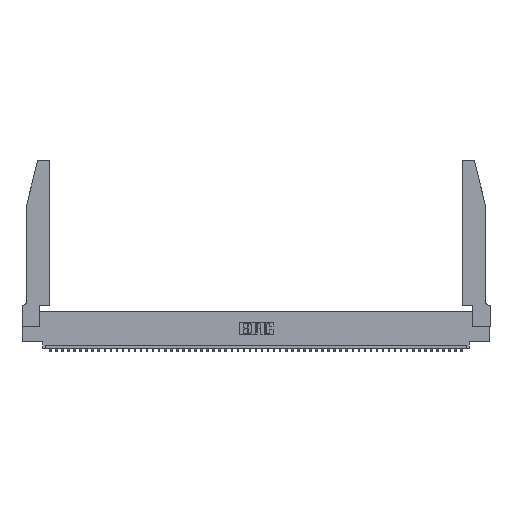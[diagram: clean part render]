
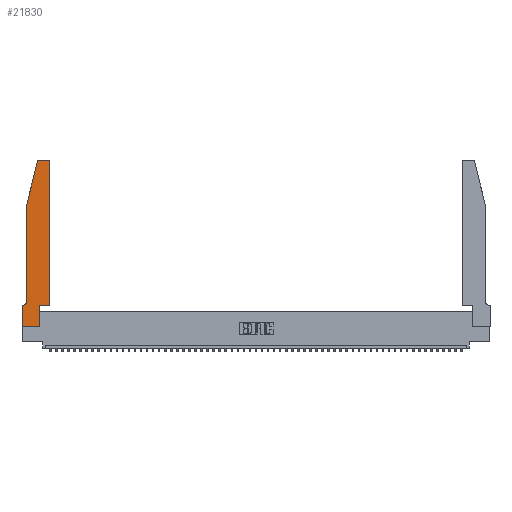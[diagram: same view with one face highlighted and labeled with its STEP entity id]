
A CAD part, top view. The second image highlights one B-rep face of the part: STEP entity #21830.
In plain terms, the highlighted planar face has unit normal (0, 0, 1).
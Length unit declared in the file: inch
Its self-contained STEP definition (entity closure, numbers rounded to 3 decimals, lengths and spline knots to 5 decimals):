
#239 = LINE ( 'NONE', #25851, #21448 ) ;
#1232 = CARTESIAN_POINT ( 'NONE',  ( 0., 0., 0.37 ) ) ;
#1386 = DIRECTION ( 'NONE',  ( 0., 0., 1. ) ) ;
#2253 = VERTEX_POINT ( 'NONE', #44497 ) ;
#3113 = VECTOR ( 'NONE', #41160, 39.37008 ) ;
#3947 = VECTOR ( 'NONE', #29542, 39.37008 ) ;
#3979 = LINE ( 'NONE', #7319, #29633 ) ;
#4258 = EDGE_CURVE ( 'NONE', #22931, #20727, #239, .T. ) ;
#4473 = ORIENTED_EDGE ( 'NONE', *, *, #10888, .T. ) ;
#4487 = CARTESIAN_POINT ( 'NONE',  ( 0.4505, 2.72, 0.37 ) ) ;
#5545 = CARTESIAN_POINT ( 'NONE',  ( 0.4205, 2.72, 0.37 ) ) ;
#6662 = EDGE_CURVE ( 'NONE', #20727, #7962, #49539, .T. ) ;
#7319 = CARTESIAN_POINT ( 'NONE',  ( 0.4505, 0.35, 0.37 ) ) ;
#7406 = VERTEX_POINT ( 'NONE', #10299 ) ;
#7962 = VERTEX_POINT ( 'NONE', #19062 ) ;
#8194 = ORIENTED_EDGE ( 'NONE', *, *, #32107, .T. ) ;
#8564 = LINE ( 'NONE', #29161, #27917 ) ;
#8769 = LINE ( 'NONE', #27854, #45506 ) ;
#9931 = EDGE_LOOP ( 'NONE', ( #43637, #41427, #31588, #38553, #4473, #43729, #26091, #50199, #17724, #44850, #39837, #8194 ) ) ;
#10299 = CARTESIAN_POINT ( 'NONE',  ( 0.25487, 2.72718, 0.37 ) ) ;
#10380 = VERTEX_POINT ( 'NONE', #24235 ) ;
#10888 = EDGE_CURVE ( 'NONE', #23437, #10380, #26225, .T. ) ;
#13756 = CARTESIAN_POINT ( 'NONE',  ( 0.0055, 0.42, 0.37 ) ) ;
#14034 = AXIS2_PLACEMENT_3D ( 'NONE', #5545, #1386, #48073 ) ;
#15065 = DIRECTION ( 'NONE',  ( 1., 0., 0. ) ) ;
#15107 = CARTESIAN_POINT ( 'NONE',  ( 0.4205, 2.75, 0.37 ) ) ;
#16115 = EDGE_CURVE ( 'NONE', #27870, #21726, #28278, .T. ) ;
#17018 = CARTESIAN_POINT ( 'NONE',  ( 0.2605, 2.75, 0.37 ) ) ;
#17303 = LINE ( 'NONE', #1232, #3947 ) ;
#17724 = ORIENTED_EDGE ( 'NONE', *, *, #6662, .T. ) ;
#18154 = AXIS2_PLACEMENT_3D ( 'NONE', #43521, #31065, #35244 ) ;
#19062 = CARTESIAN_POINT ( 'NONE',  ( 0.2865, 0.35, 0.37 ) ) ;
#19545 = DIRECTION ( 'NONE',  ( 0., 0., -1. ) ) ;
#19902 = EDGE_CURVE ( 'NONE', #7962, #46887, #3979, .T. ) ;
#20701 = AXIS2_PLACEMENT_3D ( 'NONE', #37702, #41844, #42013 ) ;
#20727 = VERTEX_POINT ( 'NONE', #30336 ) ;
#21448 = VECTOR ( 'NONE', #39375, 39.37008 ) ;
#21481 = CIRCLE ( 'NONE', #14034, 0.03 ) ;
#21726 = VERTEX_POINT ( 'NONE', #35262 ) ;
#21830 = ADVANCED_FACE ( 'NONE', ( #52040 ), #37760, .T. ) ;
#22159 = CARTESIAN_POINT ( 'NONE',  ( 0.0755, 2., 0.37 ) ) ;
#22931 = VERTEX_POINT ( 'NONE', #35348 ) ;
#23029 = AXIS2_PLACEMENT_3D ( 'NONE', #13756, #19545, #42838 ) ;
#23339 = EDGE_CURVE ( 'NONE', #7406, #36113, #36553, .T. ) ;
#23405 = EDGE_CURVE ( 'NONE', #10380, #2253, #8769, .T. ) ;
#23437 = VERTEX_POINT ( 'NONE', #53276 ) ;
#24235 = CARTESIAN_POINT ( 'NONE',  ( 0.0055, 0.35, 0.37 ) ) ;
#25851 = CARTESIAN_POINT ( 'NONE',  ( 0., 0., 0.37 ) ) ;
#26091 = ORIENTED_EDGE ( 'NONE', *, *, #33414, .T. ) ;
#26225 = CIRCLE ( 'NONE', #23029, 0.07 ) ;
#26385 = DIRECTION ( 'NONE',  ( 0., 1., 0. ) ) ;
#27424 = LINE ( 'NONE', #53063, #35157 ) ;
#27854 = CARTESIAN_POINT ( 'NONE',  ( 0.0755, 0.35, 0.37 ) ) ;
#27870 = VERTEX_POINT ( 'NONE', #15107 ) ;
#27917 = VECTOR ( 'NONE', #46079, 39.37008 ) ;
#28278 = LINE ( 'NONE', #17018, #3113 ) ;
#29161 = CARTESIAN_POINT ( 'NONE',  ( 0.0755, 2., 0.37 ) ) ;
#29542 = DIRECTION ( 'NONE',  ( 0., -1., 0. ) ) ;
#29633 = VECTOR ( 'NONE', #15065, 39.37008 ) ;
#30336 = CARTESIAN_POINT ( 'NONE',  ( 0.2865, 0., 0.37 ) ) ;
#31065 = DIRECTION ( 'NONE',  ( 0., 0., 1. ) ) ;
#31588 = ORIENTED_EDGE ( 'NONE', *, *, #23339, .T. ) ;
#32107 = EDGE_CURVE ( 'NONE', #52682, #27870, #21481, .T. ) ;
#32845 = EDGE_CURVE ( 'NONE', #36113, #23437, #8564, .T. ) ;
#33302 = VECTOR ( 'NONE', #38314, 39.37008 ) ;
#33414 = EDGE_CURVE ( 'NONE', #2253, #22931, #17303, .T. ) ;
#33609 = CARTESIAN_POINT ( 'NONE',  ( 0.2865, 0.35, 0.37 ) ) ;
#35157 = VECTOR ( 'NONE', #40979, 39.37008 ) ;
#35244 = DIRECTION ( 'NONE',  ( 1., 0., 0. ) ) ;
#35262 = CARTESIAN_POINT ( 'NONE',  ( 0.284, 2.75, 0.37 ) ) ;
#35348 = CARTESIAN_POINT ( 'NONE',  ( 0., 0., 0.37 ) ) ;
#35590 = CARTESIAN_POINT ( 'NONE',  ( 0.4505, 0.35, 0.37 ) ) ;
#36041 = VECTOR ( 'NONE', #26385, 39.37008 ) ;
#36113 = VERTEX_POINT ( 'NONE', #47512 ) ;
#36553 = LINE ( 'NONE', #22159, #33302 ) ;
#37702 = CARTESIAN_POINT ( 'NONE',  ( 0., 0.35, 0.37 ) ) ;
#37760 = PLANE ( 'NONE',  #20701 ) ;
#38314 = DIRECTION ( 'NONE',  ( -0.239, -0.971, 0. ) ) ;
#38553 = ORIENTED_EDGE ( 'NONE', *, *, #32845, .T. ) ;
#39055 = DIRECTION ( 'NONE',  ( -1., 0., 0. ) ) ;
#39375 = DIRECTION ( 'NONE',  ( 1., 0., 0. ) ) ;
#39837 = ORIENTED_EDGE ( 'NONE', *, *, #48385, .T. ) ;
#40979 = DIRECTION ( 'NONE',  ( 0., 1., 0. ) ) ;
#41160 = DIRECTION ( 'NONE',  ( -1., 0., 0. ) ) ;
#41427 = ORIENTED_EDGE ( 'NONE', *, *, #41670, .T. ) ;
#41670 = EDGE_CURVE ( 'NONE', #21726, #7406, #45752, .T. ) ;
#41844 = DIRECTION ( 'NONE',  ( 0., 0., 1. ) ) ;
#42013 = DIRECTION ( 'NONE',  ( 1., 0., 0. ) ) ;
#42838 = DIRECTION ( 'NONE',  ( -1., 0., 0. ) ) ;
#43521 = CARTESIAN_POINT ( 'NONE',  ( 0.284, 2.72, 0.37 ) ) ;
#43637 = ORIENTED_EDGE ( 'NONE', *, *, #16115, .T. ) ;
#43729 = ORIENTED_EDGE ( 'NONE', *, *, #23405, .T. ) ;
#44497 = CARTESIAN_POINT ( 'NONE',  ( 0., 0.35, 0.37 ) ) ;
#44850 = ORIENTED_EDGE ( 'NONE', *, *, #19902, .T. ) ;
#45506 = VECTOR ( 'NONE', #39055, 39.37008 ) ;
#45752 = CIRCLE ( 'NONE', #18154, 0.03 ) ;
#46079 = DIRECTION ( 'NONE',  ( 0., -1., 0. ) ) ;
#46887 = VERTEX_POINT ( 'NONE', #35590 ) ;
#47512 = CARTESIAN_POINT ( 'NONE',  ( 0.0755, 2., 0.37 ) ) ;
#48073 = DIRECTION ( 'NONE',  ( 1., 0., 0. ) ) ;
#48385 = EDGE_CURVE ( 'NONE', #46887, #52682, #27424, .T. ) ;
#49539 = LINE ( 'NONE', #33609, #36041 ) ;
#50199 = ORIENTED_EDGE ( 'NONE', *, *, #4258, .T. ) ;
#52040 = FACE_OUTER_BOUND ( 'NONE', #9931, .T. ) ;
#52682 = VERTEX_POINT ( 'NONE', #4487 ) ;
#53063 = CARTESIAN_POINT ( 'NONE',  ( 0.4505, 0.35, 0.37 ) ) ;
#53276 = CARTESIAN_POINT ( 'NONE',  ( 0.0755, 0.42, 0.37 ) ) ;
